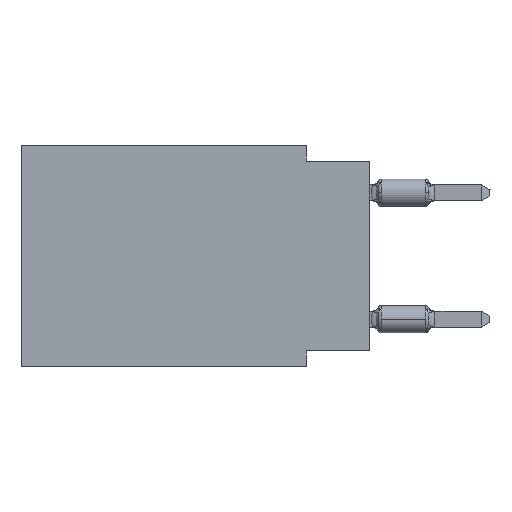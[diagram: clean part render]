
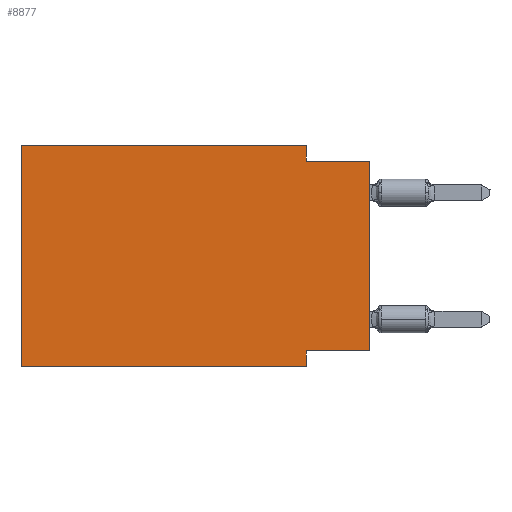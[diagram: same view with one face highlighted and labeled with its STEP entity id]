
A CAD part, left-side view. The second image highlights one B-rep face of the part: STEP entity #8877.
In plain terms, the highlighted planar face has unit normal (-1, 0, 0).
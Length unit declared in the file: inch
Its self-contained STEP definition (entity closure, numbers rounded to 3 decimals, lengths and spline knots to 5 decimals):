
#1178 = LINE ( 'NONE', #6094, #14127 ) ;
#1388 = AXIS2_PLACEMENT_3D ( 'NONE', #13035, #2602, #3658 ) ;
#1390 = EDGE_CURVE ( 'NONE', #1465, #9589, #13131, .T. ) ;
#1401 = DIRECTION ( 'NONE',  ( 0., -1., 0. ) ) ;
#1465 = VERTEX_POINT ( 'NONE', #6428 ) ;
#1788 = CARTESIAN_POINT ( 'NONE',  ( 0., 0.55, 0. ) ) ;
#1841 = ORIENTED_EDGE ( 'NONE', *, *, #5150, .F. ) ;
#2289 = VERTEX_POINT ( 'NONE', #11179 ) ;
#2523 = EDGE_CURVE ( 'NONE', #9589, #13709, #4866, .T. ) ;
#2548 = ORIENTED_EDGE ( 'NONE', *, *, #2523, .F. ) ;
#2602 = DIRECTION ( 'NONE',  ( 1., 0., 0. ) ) ;
#2760 = CARTESIAN_POINT ( 'NONE',  ( 0., 0., -0.025 ) ) ;
#2848 = VECTOR ( 'NONE', #11933, 39.37008 ) ;
#2944 = PLANE ( 'NONE',  #1388 ) ;
#3169 = VERTEX_POINT ( 'NONE', #13658 ) ;
#3350 = ORIENTED_EDGE ( 'NONE', *, *, #8585, .F. ) ;
#3658 = DIRECTION ( 'NONE',  ( 0., 0., -1. ) ) ;
#4283 = CARTESIAN_POINT ( 'NONE',  ( 0., 0., 0. ) ) ;
#4502 = CARTESIAN_POINT ( 'NONE',  ( 0., 0.1, -0.025 ) ) ;
#4546 = VECTOR ( 'NONE', #7495, 39.37008 ) ;
#4548 = ORIENTED_EDGE ( 'NONE', *, *, #12891, .F. ) ;
#4672 = VECTOR ( 'NONE', #4781, 39.37008 ) ;
#4781 = DIRECTION ( 'NONE',  ( 0., 0., -1. ) ) ;
#4866 = LINE ( 'NONE', #14217, #2848 ) ;
#5077 = ORIENTED_EDGE ( 'NONE', *, *, #12392, .F. ) ;
#5150 = EDGE_CURVE ( 'NONE', #12240, #11484, #14142, .T. ) ;
#5280 = LINE ( 'NONE', #4283, #5695 ) ;
#5695 = VECTOR ( 'NONE', #9985, 39.37008 ) ;
#6094 = CARTESIAN_POINT ( 'NONE',  ( 0., 0.55, -0.35 ) ) ;
#6126 = DIRECTION ( 'NONE',  ( 0., 0., -1. ) ) ;
#6205 = CARTESIAN_POINT ( 'NONE',  ( 0., 0.1, 0. ) ) ;
#6287 = CARTESIAN_POINT ( 'NONE',  ( 0., 0.55, 0. ) ) ;
#6428 = CARTESIAN_POINT ( 'NONE',  ( 0., 0.1, 0. ) ) ;
#7341 = VECTOR ( 'NONE', #8232, 39.37008 ) ;
#7495 = DIRECTION ( 'NONE',  ( 0., 0., 1. ) ) ;
#8232 = DIRECTION ( 'NONE',  ( 0., 1., 0. ) ) ;
#8585 = EDGE_CURVE ( 'NONE', #2289, #8891, #14471, .T. ) ;
#8877 = ADVANCED_FACE ( 'NONE', ( #9382 ), #2944, .F. ) ;
#8891 = VERTEX_POINT ( 'NONE', #11878 ) ;
#9333 = EDGE_LOOP ( 'NONE', ( #12124, #2548, #12147, #4548, #3350, #14503, #5077, #1841 ) ) ;
#9372 = CARTESIAN_POINT ( 'NONE',  ( 0., 0., -0.325 ) ) ;
#9382 = FACE_OUTER_BOUND ( 'NONE', #9333, .T. ) ;
#9563 = DIRECTION ( 'NONE',  ( 0., -1., 0. ) ) ;
#9589 = VERTEX_POINT ( 'NONE', #4502 ) ;
#9985 = DIRECTION ( 'NONE',  ( 0., 0., 1. ) ) ;
#10567 = CARTESIAN_POINT ( 'NONE',  ( 0., 0.1, -0.35 ) ) ;
#11113 = VECTOR ( 'NONE', #6126, 39.37008 ) ;
#11179 = CARTESIAN_POINT ( 'NONE',  ( 0., 0.55, -0.35 ) ) ;
#11484 = VERTEX_POINT ( 'NONE', #12520 ) ;
#11630 = LINE ( 'NONE', #10567, #4672 ) ;
#11878 = CARTESIAN_POINT ( 'NONE',  ( 0., 0.55, 0. ) ) ;
#11933 = DIRECTION ( 'NONE',  ( 0., -1., 0. ) ) ;
#11948 = EDGE_CURVE ( 'NONE', #2289, #3169, #1178, .T. ) ;
#12124 = ORIENTED_EDGE ( 'NONE', *, *, #15002, .T. ) ;
#12147 = ORIENTED_EDGE ( 'NONE', *, *, #1390, .F. ) ;
#12240 = VERTEX_POINT ( 'NONE', #12558 ) ;
#12392 = EDGE_CURVE ( 'NONE', #11484, #3169, #11630, .T. ) ;
#12520 = CARTESIAN_POINT ( 'NONE',  ( 0., 0.1, -0.325 ) ) ;
#12558 = CARTESIAN_POINT ( 'NONE',  ( 0., 0., -0.325 ) ) ;
#12891 = EDGE_CURVE ( 'NONE', #8891, #1465, #12994, .T. ) ;
#12994 = LINE ( 'NONE', #6287, #14153 ) ;
#13035 = CARTESIAN_POINT ( 'NONE',  ( 0., 0.55, 0. ) ) ;
#13131 = LINE ( 'NONE', #6205, #11113 ) ;
#13658 = CARTESIAN_POINT ( 'NONE',  ( 0., 0.1, -0.35 ) ) ;
#13709 = VERTEX_POINT ( 'NONE', #2760 ) ;
#14127 = VECTOR ( 'NONE', #1401, 39.37008 ) ;
#14142 = LINE ( 'NONE', #9372, #7341 ) ;
#14153 = VECTOR ( 'NONE', #9563, 39.37008 ) ;
#14217 = CARTESIAN_POINT ( 'NONE',  ( 0., 0., -0.025 ) ) ;
#14471 = LINE ( 'NONE', #1788, #4546 ) ;
#14503 = ORIENTED_EDGE ( 'NONE', *, *, #11948, .T. ) ;
#15002 = EDGE_CURVE ( 'NONE', #12240, #13709, #5280, .T. ) ;
